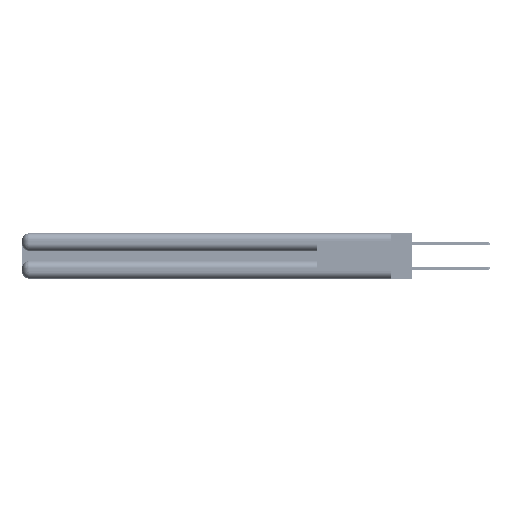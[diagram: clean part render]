
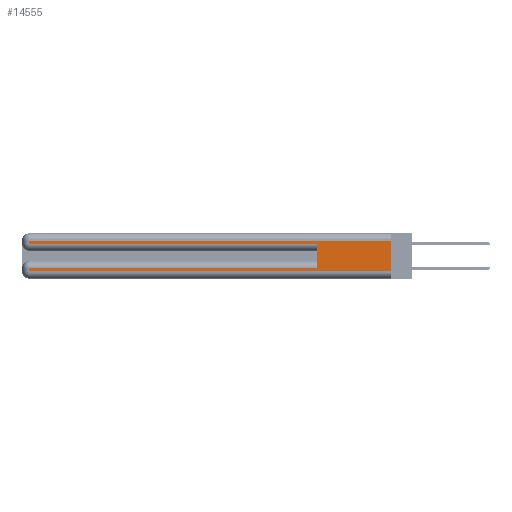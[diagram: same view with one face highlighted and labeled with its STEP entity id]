
A CAD part, left-side view. The second image highlights one B-rep face of the part: STEP entity #14555.
In plain terms, the highlighted planar face has unit normal (-1, 0, 0).
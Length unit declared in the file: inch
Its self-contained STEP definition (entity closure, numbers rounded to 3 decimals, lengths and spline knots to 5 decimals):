
#108 = CARTESIAN_POINT ( 'NONE',  ( 0., 0., 0.37 ) ) ;
#1312 = EDGE_CURVE ( 'NONE', #13527, #52148, #34065, .T. ) ;
#1446 = VERTEX_POINT ( 'NONE', #3667 ) ;
#1937 = VECTOR ( 'NONE', #20302, 39.37008 ) ;
#2254 = CARTESIAN_POINT ( 'NONE',  ( 0., 2.94, 0.37 ) ) ;
#3667 = CARTESIAN_POINT ( 'NONE',  ( 0., 0., 0.06 ) ) ;
#4092 = VECTOR ( 'NONE', #36826, 39.37008 ) ;
#4591 = CARTESIAN_POINT ( 'NONE',  ( 0., 0.6, 0.085 ) ) ;
#5100 = LINE ( 'NONE', #20688, #39282 ) ;
#5413 = LINE ( 'NONE', #14409, #34022 ) ;
#6123 = LINE ( 'NONE', #30437, #7518 ) ;
#6502 = CARTESIAN_POINT ( 'NONE',  ( 0., 2.94, 0.31 ) ) ;
#6750 = DIRECTION ( 'NONE',  ( 0., 0., -1. ) ) ;
#7518 = VECTOR ( 'NONE', #47789, 39.37008 ) ;
#8900 = ORIENTED_EDGE ( 'NONE', *, *, #13625, .T. ) ;
#10290 = AXIS2_PLACEMENT_3D ( 'NONE', #108, #33088, #31142 ) ;
#12656 = ORIENTED_EDGE ( 'NONE', *, *, #43134, .T. ) ;
#13527 = VERTEX_POINT ( 'NONE', #41930 ) ;
#13589 = VERTEX_POINT ( 'NONE', #46428 ) ;
#13625 = EDGE_CURVE ( 'NONE', #52148, #13589, #6123, .T. ) ;
#14409 = CARTESIAN_POINT ( 'NONE',  ( 0., 0., 0.285 ) ) ;
#14555 = ADVANCED_FACE ( 'NONE', ( #35331 ), #22183, .F. ) ;
#14558 = VERTEX_POINT ( 'NONE', #4591 ) ;
#15012 = DIRECTION ( 'NONE',  ( 0., 0., -1. ) ) ;
#15789 = EDGE_CURVE ( 'NONE', #14558, #36207, #5100, .T. ) ;
#16355 = LINE ( 'NONE', #50879, #40681 ) ;
#16566 = CARTESIAN_POINT ( 'NONE',  ( 0., 0., 0.31 ) ) ;
#20302 = DIRECTION ( 'NONE',  ( 0., 1., 0. ) ) ;
#20688 = CARTESIAN_POINT ( 'NONE',  ( 0., 0.6, 0.145 ) ) ;
#22123 = EDGE_CURVE ( 'NONE', #47899, #1446, #33601, .T. ) ;
#22183 = PLANE ( 'NONE',  #10290 ) ;
#23062 = EDGE_CURVE ( 'NONE', #25120, #47899, #53837, .T. ) ;
#23773 = DIRECTION ( 'NONE',  ( 0., -1., 0. ) ) ;
#24329 = EDGE_CURVE ( 'NONE', #14558, #25120, #40329, .T. ) ;
#25120 = VERTEX_POINT ( 'NONE', #25477 ) ;
#25217 = CARTESIAN_POINT ( 'NONE',  ( 0., 0., 0.06 ) ) ;
#25477 = CARTESIAN_POINT ( 'NONE',  ( 0., 2.94, 0.085 ) ) ;
#29633 = DIRECTION ( 'NONE',  ( 0., 0., 1. ) ) ;
#29820 = ORIENTED_EDGE ( 'NONE', *, *, #1312, .T. ) ;
#30095 = ORIENTED_EDGE ( 'NONE', *, *, #23062, .T. ) ;
#30437 = CARTESIAN_POINT ( 'NONE',  ( 0., 2.94, 0.37 ) ) ;
#30515 = ORIENTED_EDGE ( 'NONE', *, *, #24329, .T. ) ;
#31142 = DIRECTION ( 'NONE',  ( 0., 0., -1. ) ) ;
#31608 = ORIENTED_EDGE ( 'NONE', *, *, #15789, .F. ) ;
#33088 = DIRECTION ( 'NONE',  ( 1., 0., 0. ) ) ;
#33601 = LINE ( 'NONE', #25217, #57413 ) ;
#33778 = DIRECTION ( 'NONE',  ( 0., -1., 0. ) ) ;
#34022 = VECTOR ( 'NONE', #23773, 39.37008 ) ;
#34065 = LINE ( 'NONE', #16566, #1937 ) ;
#34665 = CARTESIAN_POINT ( 'NONE',  ( 0., 0.6, 0.285 ) ) ;
#35331 = FACE_OUTER_BOUND ( 'NONE', #36694, .T. ) ;
#35368 = ORIENTED_EDGE ( 'NONE', *, *, #35838, .F. ) ;
#35838 = EDGE_CURVE ( 'NONE', #13527, #1446, #16355, .T. ) ;
#36207 = VERTEX_POINT ( 'NONE', #34665 ) ;
#36694 = EDGE_LOOP ( 'NONE', ( #35368, #29820, #8900, #12656, #31608, #30515, #30095, #51809 ) ) ;
#36826 = DIRECTION ( 'NONE',  ( 0., 1., 0. ) ) ;
#39282 = VECTOR ( 'NONE', #29633, 39.37008 ) ;
#40329 = LINE ( 'NONE', #45190, #4092 ) ;
#40681 = VECTOR ( 'NONE', #15012, 39.37008 ) ;
#41930 = CARTESIAN_POINT ( 'NONE',  ( 0., 0., 0.31 ) ) ;
#43134 = EDGE_CURVE ( 'NONE', #13589, #36207, #5413, .T. ) ;
#45190 = CARTESIAN_POINT ( 'NONE',  ( 0., 0., 0.085 ) ) ;
#46428 = CARTESIAN_POINT ( 'NONE',  ( 0., 2.94, 0.285 ) ) ;
#47789 = DIRECTION ( 'NONE',  ( 0., 0., -1. ) ) ;
#47899 = VERTEX_POINT ( 'NONE', #49107 ) ;
#48247 = VECTOR ( 'NONE', #6750, 39.37008 ) ;
#49107 = CARTESIAN_POINT ( 'NONE',  ( 0., 2.94, 0.06 ) ) ;
#50879 = CARTESIAN_POINT ( 'NONE',  ( 0., 0., 0.37 ) ) ;
#51809 = ORIENTED_EDGE ( 'NONE', *, *, #22123, .T. ) ;
#52148 = VERTEX_POINT ( 'NONE', #6502 ) ;
#53837 = LINE ( 'NONE', #2254, #48247 ) ;
#57413 = VECTOR ( 'NONE', #33778, 39.37008 ) ;
